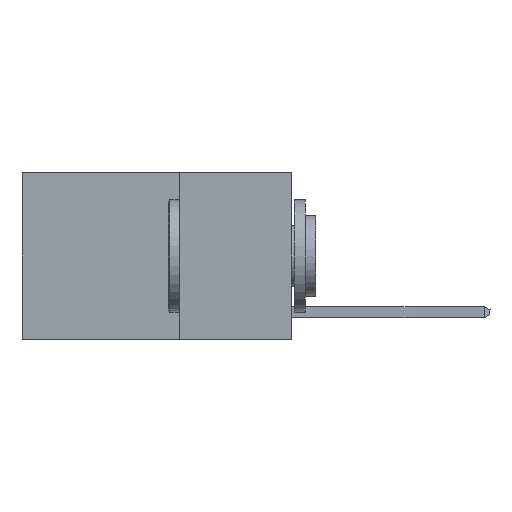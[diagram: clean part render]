
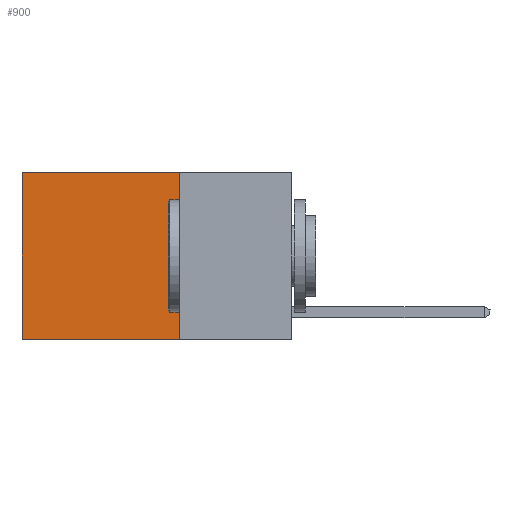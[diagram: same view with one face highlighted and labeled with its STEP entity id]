
A CAD part, left-side view. The second image highlights one B-rep face of the part: STEP entity #900.
In plain terms, the highlighted planar face has unit normal (-1, 0, 0).
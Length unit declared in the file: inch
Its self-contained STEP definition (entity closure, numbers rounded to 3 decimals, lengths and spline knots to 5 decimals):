
#422 = CARTESIAN_POINT ( 'NONE',  ( 0.2625, 0.25, -0.37 ) ) ;
#900 = ADVANCED_FACE ( 'NONE', ( #2593 ), #20359, .F. ) ;
#2485 = CARTESIAN_POINT ( 'NONE',  ( 0.2625, 0.25, 0. ) ) ;
#2593 = FACE_OUTER_BOUND ( 'NONE', #27852, .T. ) ;
#2649 = EDGE_CURVE ( 'NONE', #4511, #8892, #9858, .T. ) ;
#2680 = VECTOR ( 'NONE', #21004, 39.37008 ) ;
#2700 = DIRECTION ( 'NONE',  ( 0., 0., -1. ) ) ;
#2827 = VECTOR ( 'NONE', #20440, 39.37008 ) ;
#2863 = DIRECTION ( 'NONE',  ( 0., 0., -1. ) ) ;
#4511 = VERTEX_POINT ( 'NONE', #19453 ) ;
#5017 = CARTESIAN_POINT ( 'NONE',  ( 0.2625, 0.25, 0. ) ) ;
#5255 = EDGE_CURVE ( 'NONE', #14842, #22638, #12156, .T. ) ;
#7616 = ORIENTED_EDGE ( 'NONE', *, *, #2649, .T. ) ;
#8172 = LINE ( 'NONE', #5017, #15615 ) ;
#8247 = EDGE_CURVE ( 'NONE', #8892, #22638, #15554, .T. ) ;
#8892 = VERTEX_POINT ( 'NONE', #26540 ) ;
#9858 = LINE ( 'NONE', #2485, #2827 ) ;
#12156 = LINE ( 'NONE', #422, #2680 ) ;
#14842 = VERTEX_POINT ( 'NONE', #28631 ) ;
#15554 = LINE ( 'NONE', #16772, #27195 ) ;
#15615 = VECTOR ( 'NONE', #2863, 39.37008 ) ;
#16291 = DIRECTION ( 'NONE',  ( 1., 0., 0. ) ) ;
#16772 = CARTESIAN_POINT ( 'NONE',  ( 0.2625, 0.6, 0. ) ) ;
#19453 = CARTESIAN_POINT ( 'NONE',  ( 0.2625, 0.25, 0. ) ) ;
#20269 = CARTESIAN_POINT ( 'NONE',  ( 0.2625, 0.25, 0. ) ) ;
#20359 = PLANE ( 'NONE',  #23207 ) ;
#20440 = DIRECTION ( 'NONE',  ( 0., 1., 0. ) ) ;
#21004 = DIRECTION ( 'NONE',  ( 0., 1., 0. ) ) ;
#21189 = CARTESIAN_POINT ( 'NONE',  ( 0.2625, 0.6, -0.37 ) ) ;
#22063 = ORIENTED_EDGE ( 'NONE', *, *, #8247, .T. ) ;
#22638 = VERTEX_POINT ( 'NONE', #21189 ) ;
#23207 = AXIS2_PLACEMENT_3D ( 'NONE', #20269, #16291, #2700 ) ;
#23772 = ORIENTED_EDGE ( 'NONE', *, *, #5255, .F. ) ;
#25556 = DIRECTION ( 'NONE',  ( 0., 0., -1. ) ) ;
#26167 = EDGE_CURVE ( 'NONE', #4511, #14842, #8172, .T. ) ;
#26540 = CARTESIAN_POINT ( 'NONE',  ( 0.2625, 0.6, 0. ) ) ;
#27195 = VECTOR ( 'NONE', #25556, 39.37008 ) ;
#27852 = EDGE_LOOP ( 'NONE', ( #22063, #23772, #28538, #7616 ) ) ;
#28538 = ORIENTED_EDGE ( 'NONE', *, *, #26167, .F. ) ;
#28631 = CARTESIAN_POINT ( 'NONE',  ( 0.2625, 0.25, -0.37 ) ) ;
